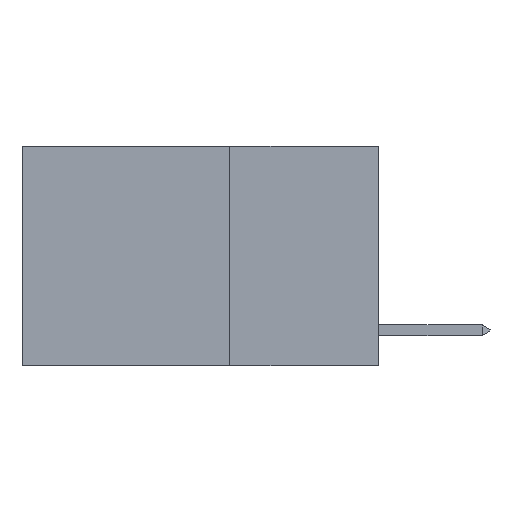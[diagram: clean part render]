
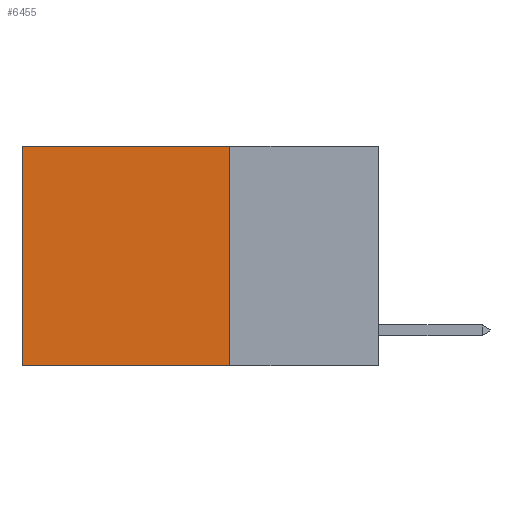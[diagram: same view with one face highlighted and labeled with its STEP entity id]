
A CAD part, left-side view. The second image highlights one B-rep face of the part: STEP entity #6455.
In plain terms, the highlighted planar face has unit normal (-1, 0, 0).
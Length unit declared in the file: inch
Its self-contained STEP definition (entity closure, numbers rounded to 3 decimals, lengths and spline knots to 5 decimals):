
#477 = CARTESIAN_POINT ( 'NONE',  ( 0.2625, 0.6, 0. ) ) ;
#564 = DIRECTION ( 'NONE',  ( 0., 0., -1. ) ) ;
#988 = CARTESIAN_POINT ( 'NONE',  ( 0.2625, 0.25, 0. ) ) ;
#1254 = LINE ( 'NONE', #13775, #7088 ) ;
#2029 = ORIENTED_EDGE ( 'NONE', *, *, #7054, .F. ) ;
#2463 = VECTOR ( 'NONE', #6404, 39.37008 ) ;
#2802 = DIRECTION ( 'NONE',  ( 0., 1., 0. ) ) ;
#3279 = DIRECTION ( 'NONE',  ( 1., 0., 0. ) ) ;
#3454 = CARTESIAN_POINT ( 'NONE',  ( 0.2625, 0.25, 0. ) ) ;
#4204 = VERTEX_POINT ( 'NONE', #7204 ) ;
#4432 = AXIS2_PLACEMENT_3D ( 'NONE', #3454, #3279, #8995 ) ;
#4854 = CARTESIAN_POINT ( 'NONE',  ( 0.2625, 0.25, -0.37 ) ) ;
#5484 = VERTEX_POINT ( 'NONE', #6011 ) ;
#6011 = CARTESIAN_POINT ( 'NONE',  ( 0.2625, 0.25, -0.37 ) ) ;
#6404 = DIRECTION ( 'NONE',  ( 0., 1., 0. ) ) ;
#6455 = ADVANCED_FACE ( 'NONE', ( #7533 ), #13066, .F. ) ;
#7003 = EDGE_LOOP ( 'NONE', ( #16272, #11331, #2029, #14546 ) ) ;
#7054 = EDGE_CURVE ( 'NONE', #14636, #5484, #17485, .T. ) ;
#7088 = VECTOR ( 'NONE', #2802, 39.37008 ) ;
#7204 = CARTESIAN_POINT ( 'NONE',  ( 0.2625, 0.6, 0. ) ) ;
#7377 = VECTOR ( 'NONE', #9058, 39.37008 ) ;
#7492 = EDGE_CURVE ( 'NONE', #5484, #17852, #9134, .T. ) ;
#7533 = FACE_OUTER_BOUND ( 'NONE', #7003, .T. ) ;
#8440 = EDGE_CURVE ( 'NONE', #14636, #4204, #1254, .T. ) ;
#8946 = EDGE_CURVE ( 'NONE', #4204, #17852, #16981, .T. ) ;
#8995 = DIRECTION ( 'NONE',  ( 0., 0., -1. ) ) ;
#9058 = DIRECTION ( 'NONE',  ( 0., 0., -1. ) ) ;
#9134 = LINE ( 'NONE', #4854, #2463 ) ;
#11331 = ORIENTED_EDGE ( 'NONE', *, *, #7492, .F. ) ;
#13066 = PLANE ( 'NONE',  #4432 ) ;
#13748 = CARTESIAN_POINT ( 'NONE',  ( 0.2625, 0.6, -0.37 ) ) ;
#13775 = CARTESIAN_POINT ( 'NONE',  ( 0.2625, 0.25, 0. ) ) ;
#14359 = VECTOR ( 'NONE', #564, 39.37008 ) ;
#14365 = CARTESIAN_POINT ( 'NONE',  ( 0.2625, 0.25, 0. ) ) ;
#14546 = ORIENTED_EDGE ( 'NONE', *, *, #8440, .T. ) ;
#14636 = VERTEX_POINT ( 'NONE', #14365 ) ;
#16272 = ORIENTED_EDGE ( 'NONE', *, *, #8946, .T. ) ;
#16981 = LINE ( 'NONE', #477, #14359 ) ;
#17485 = LINE ( 'NONE', #988, #7377 ) ;
#17852 = VERTEX_POINT ( 'NONE', #13748 ) ;
